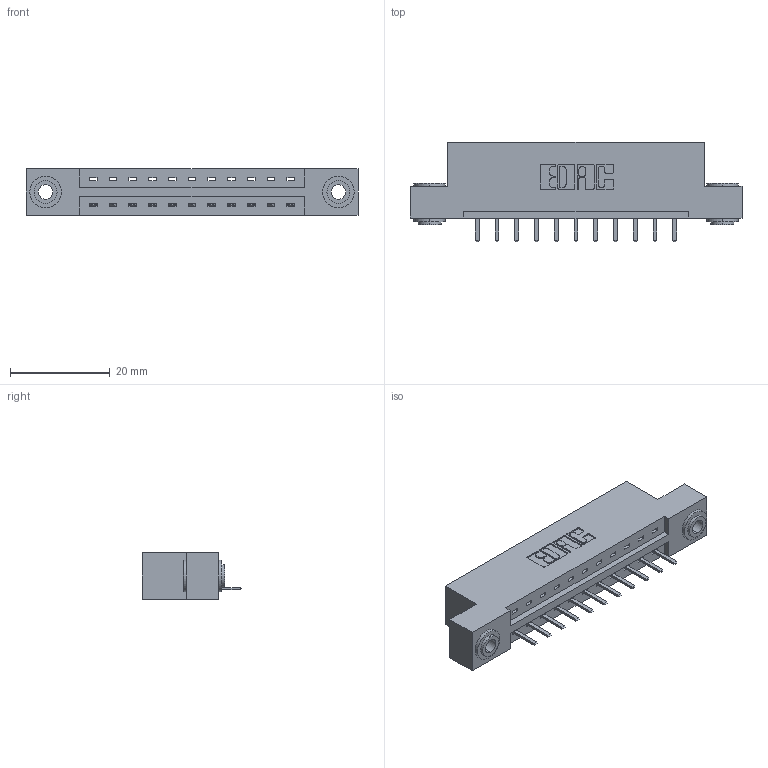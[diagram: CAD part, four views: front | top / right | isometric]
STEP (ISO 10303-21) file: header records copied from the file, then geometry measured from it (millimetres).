
FILE_DESCRIPTION (( 'STEP AP203' ), '1' );
FILE_NAME ('337-011-520-103.STEP', '2019-09-27T22:16:27', ( '' ), ( '' ), 'SwSTEP 2.0', 'SolidWorks 2016', '' );
FILE_SCHEMA (( 'CONFIG_CONTROL_DESIGN' ));
Length unit declared in the file: inch
Products named in the file (4): 337-011-520-103; 337 Part_Flush Mounting Lugs - 0.156 Dia-TH; 345-250-002_345-250-002-102; 345-292-001_345-293-120
Assembly tree (14 placements, depth 2):
  337-011-520-103
    337 Part_Flush Mounting Lugs - 0.156 Dia-TH
    345-292-001_345-293-120  x11
    345-250-002_345-250-002-102  x2
Bounding box: 66.6 x 20.02 x 9.4 mm (x, y, z)
Volume: 6521.6 mm3; surface area: 6685.9 mm2
Topology: 14 solids, 14 shells, 878 faces, 2543 edges, 1662 vertices
Faces by surface type: plane 608, cylinder 262, cone 8
Entity records: 12950 total; most frequent: CARTESIAN_POINT 2242, ORIENTED_EDGE 2170, DIRECTION 1973, EDGE_CURVE 1085, LINE 929, VECTOR 929, VERTEX_POINT 718, AXIS2_PLACEMENT_3D 522
